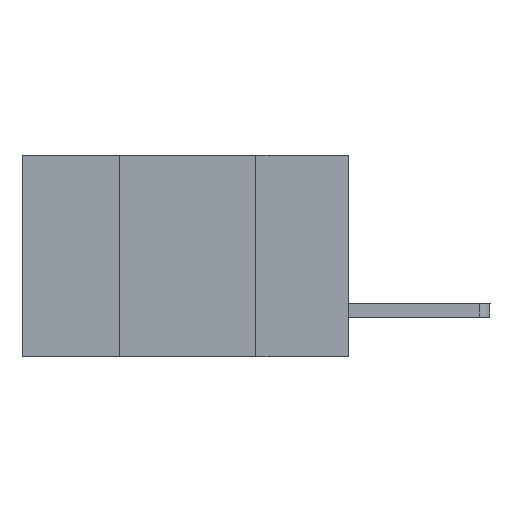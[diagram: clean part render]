
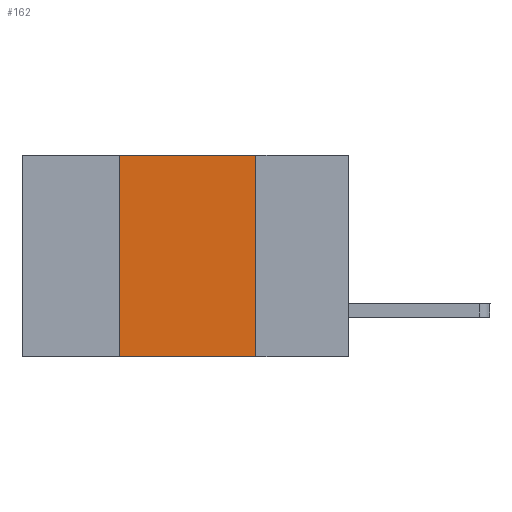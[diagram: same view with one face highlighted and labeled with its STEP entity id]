
A CAD part, left-side view. The second image highlights one B-rep face of the part: STEP entity #162.
In plain terms, the highlighted planar face has unit normal (-1, 0, 0).
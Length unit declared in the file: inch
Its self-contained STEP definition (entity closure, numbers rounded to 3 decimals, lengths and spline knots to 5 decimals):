
#28 = EDGE_CURVE ( 'NONE', #3702, #4056, #4985, .T. ) ;
#51 = ORIENTED_EDGE ( 'NONE', *, *, #5958, .F. ) ;
#162 = ADVANCED_FACE ( 'NONE', ( #1497 ), #7853, .F. ) ;
#509 = LINE ( 'NONE', #3011, #7424 ) ;
#553 = EDGE_CURVE ( 'NONE', #5242, #10004, #594, .T. ) ;
#584 = DIRECTION ( 'NONE',  ( 0., 0., -1. ) ) ;
#594 = LINE ( 'NONE', #1053, #8927 ) ;
#780 = AXIS2_PLACEMENT_3D ( 'NONE', #3810, #9443, #2237 ) ;
#1053 = CARTESIAN_POINT ( 'NONE',  ( 0., 0.6, 0. ) ) ;
#1497 = FACE_OUTER_BOUND ( 'NONE', #7761, .T. ) ;
#1990 = DIRECTION ( 'NONE',  ( 0., -1., 0. ) ) ;
#2111 = DIRECTION ( 'NONE',  ( 0., 0., 1. ) ) ;
#2133 = LINE ( 'NONE', #5368, #8702 ) ;
#2237 = DIRECTION ( 'NONE',  ( 0., 0., -1. ) ) ;
#2444 = ORIENTED_EDGE ( 'NONE', *, *, #553, .F. ) ;
#2544 = CARTESIAN_POINT ( 'NONE',  ( 0., 0.17, -0.37 ) ) ;
#3011 = CARTESIAN_POINT ( 'NONE',  ( 0., 0.42, 0. ) ) ;
#3702 = VERTEX_POINT ( 'NONE', #5544 ) ;
#3810 = CARTESIAN_POINT ( 'NONE',  ( 0., 0.6, 0. ) ) ;
#3903 = VECTOR ( 'NONE', #1990, 39.37008 ) ;
#4056 = VERTEX_POINT ( 'NONE', #2544 ) ;
#4258 = DIRECTION ( 'NONE',  ( 0., -1., 0. ) ) ;
#4498 = CARTESIAN_POINT ( 'NONE',  ( 0., 0.6, -0.37 ) ) ;
#4900 = ORIENTED_EDGE ( 'NONE', *, *, #28, .T. ) ;
#4985 = LINE ( 'NONE', #4498, #3903 ) ;
#5242 = VERTEX_POINT ( 'NONE', #8314 ) ;
#5368 = CARTESIAN_POINT ( 'NONE',  ( 0., 0.17, 0. ) ) ;
#5544 = CARTESIAN_POINT ( 'NONE',  ( 0., 0.42, -0.37 ) ) ;
#5958 = EDGE_CURVE ( 'NONE', #10004, #4056, #2133, .T. ) ;
#6258 = EDGE_CURVE ( 'NONE', #3702, #5242, #509, .T. ) ;
#6470 = ORIENTED_EDGE ( 'NONE', *, *, #6258, .F. ) ;
#6825 = CARTESIAN_POINT ( 'NONE',  ( 0., 0.17, 0. ) ) ;
#7424 = VECTOR ( 'NONE', #2111, 39.37008 ) ;
#7761 = EDGE_LOOP ( 'NONE', ( #51, #2444, #6470, #4900 ) ) ;
#7853 = PLANE ( 'NONE',  #780 ) ;
#8314 = CARTESIAN_POINT ( 'NONE',  ( 0., 0.42, 0. ) ) ;
#8702 = VECTOR ( 'NONE', #584, 39.37008 ) ;
#8927 = VECTOR ( 'NONE', #4258, 39.37008 ) ;
#9443 = DIRECTION ( 'NONE',  ( 1., 0., 0. ) ) ;
#10004 = VERTEX_POINT ( 'NONE', #6825 ) ;
